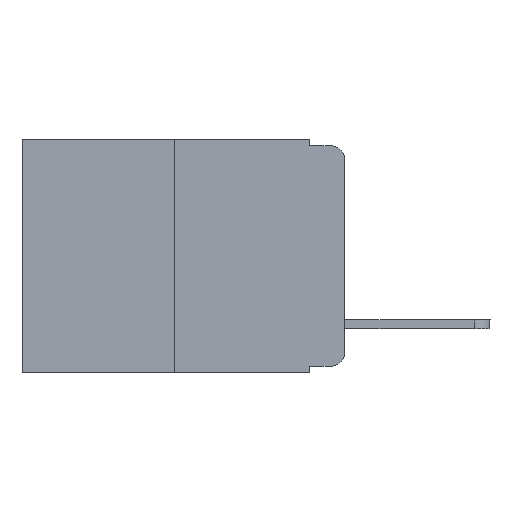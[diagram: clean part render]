
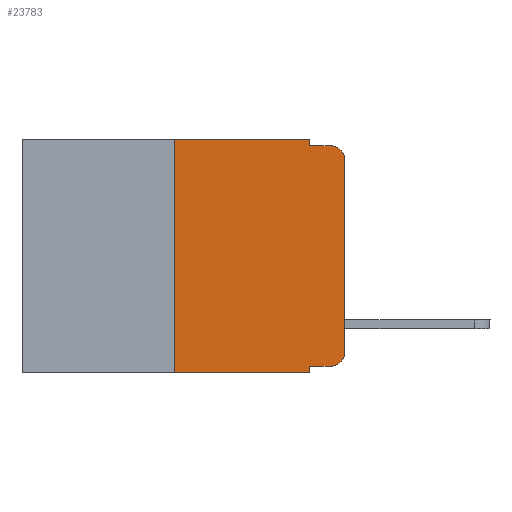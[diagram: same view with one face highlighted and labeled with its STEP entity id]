
A CAD part, left-side view. The second image highlights one B-rep face of the part: STEP entity #23783.
In plain terms, the highlighted planar face has unit normal (-1, 0, 0).
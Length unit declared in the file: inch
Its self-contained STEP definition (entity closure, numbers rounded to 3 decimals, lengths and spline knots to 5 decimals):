
#122 = CARTESIAN_POINT ( 'NONE',  ( 0., 0.25, -0.343 ) ) ;
#177 = ORIENTED_EDGE ( 'NONE', *, *, #20102, .F. ) ;
#269 = AXIS2_PLACEMENT_3D ( 'NONE', #5759, #7558, #11463 ) ;
#439 = DIRECTION ( 'NONE',  ( 0., 0., -1. ) ) ;
#513 = CARTESIAN_POINT ( 'NONE',  ( 0., 0.051, 0. ) ) ;
#537 = DIRECTION ( 'NONE',  ( 0., -1., 0. ) ) ;
#1593 = VECTOR ( 'NONE', #10630, 39.37008 ) ;
#1850 = VERTEX_POINT ( 'NONE', #20672 ) ;
#1998 = DIRECTION ( 'NONE',  ( 0., 0., -1. ) ) ;
#2379 = VERTEX_POINT ( 'NONE', #18623 ) ;
#2406 = ORIENTED_EDGE ( 'NONE', *, *, #16903, .T. ) ;
#3853 = VERTEX_POINT ( 'NONE', #6978 ) ;
#4086 = LINE ( 'NONE', #17225, #21577 ) ;
#4166 = ORIENTED_EDGE ( 'NONE', *, *, #22114, .F. ) ;
#4589 = LINE ( 'NONE', #5526, #17070 ) ;
#4627 = DIRECTION ( 'NONE',  ( 0., -1., 0. ) ) ;
#4696 = EDGE_LOOP ( 'NONE', ( #5741, #11026, #177, #17013, #11236, #5435, #10007, #4166, #2406, #10488 ) ) ;
#5435 = ORIENTED_EDGE ( 'NONE', *, *, #19730, .F. ) ;
#5526 = CARTESIAN_POINT ( 'NONE',  ( 0., 0., 0. ) ) ;
#5741 = ORIENTED_EDGE ( 'NONE', *, *, #14274, .T. ) ;
#5759 = CARTESIAN_POINT ( 'NONE',  ( 0., 0.473, 0. ) ) ;
#5960 = DIRECTION ( 'NONE',  ( 0., 0., -1. ) ) ;
#6978 = CARTESIAN_POINT ( 'NONE',  ( 0., 0.051, -0.343 ) ) ;
#7090 = VERTEX_POINT ( 'NONE', #17525 ) ;
#7213 = VERTEX_POINT ( 'NONE', #21332 ) ;
#7558 = DIRECTION ( 'NONE',  ( 1., 0., 0. ) ) ;
#7773 = LINE ( 'NONE', #12404, #1593 ) ;
#7803 = PLANE ( 'NONE',  #269 ) ;
#8147 = CARTESIAN_POINT ( 'NONE',  ( 0., 0.473, 0. ) ) ;
#8758 = LINE ( 'NONE', #8147, #18013 ) ;
#8973 = DIRECTION ( 'NONE',  ( -1., 0., 0. ) ) ;
#9135 = LINE ( 'NONE', #17227, #18108 ) ;
#9773 = CIRCLE ( 'NONE', #20121, 0.02 ) ;
#10007 = ORIENTED_EDGE ( 'NONE', *, *, #23182, .T. ) ;
#10488 = ORIENTED_EDGE ( 'NONE', *, *, #12250, .T. ) ;
#10630 = DIRECTION ( 'NONE',  ( 0., 0., 1. ) ) ;
#11026 = ORIENTED_EDGE ( 'NONE', *, *, #17869, .T. ) ;
#11236 = ORIENTED_EDGE ( 'NONE', *, *, #18863, .F. ) ;
#11435 = DIRECTION ( 'NONE',  ( -1., 0., 0. ) ) ;
#11463 = DIRECTION ( 'NONE',  ( 0., 0., -1. ) ) ;
#11502 = CARTESIAN_POINT ( 'NONE',  ( 0., 0.051, 0. ) ) ;
#11730 = DIRECTION ( 'NONE',  ( 0., -1., 0. ) ) ;
#12250 = EDGE_CURVE ( 'NONE', #2379, #14583, #9773, .T. ) ;
#12393 = CARTESIAN_POINT ( 'NONE',  ( 0., 0.051, -0.333 ) ) ;
#12404 = CARTESIAN_POINT ( 'NONE',  ( 0., 0.25, 0. ) ) ;
#13252 = VERTEX_POINT ( 'NONE', #513 ) ;
#13514 = CARTESIAN_POINT ( 'NONE',  ( 0., 0.02, -0.01 ) ) ;
#14272 = CARTESIAN_POINT ( 'NONE',  ( 0., 0.02, -0.03 ) ) ;
#14274 = EDGE_CURVE ( 'NONE', #14583, #7213, #4589, .T. ) ;
#14583 = VERTEX_POINT ( 'NONE', #19643 ) ;
#14585 = CIRCLE ( 'NONE', #17061, 0.02 ) ;
#14718 = DIRECTION ( 'NONE',  ( 0., 0., 1. ) ) ;
#14923 = VECTOR ( 'NONE', #537, 39.37008 ) ;
#15267 = LINE ( 'NONE', #11502, #21446 ) ;
#15287 = VECTOR ( 'NONE', #4627, 39.37008 ) ;
#15658 = DIRECTION ( 'NONE',  ( 0., -1., 0. ) ) ;
#16164 = LINE ( 'NONE', #20034, #15287 ) ;
#16903 = EDGE_CURVE ( 'NONE', #18139, #2379, #17539, .T. ) ;
#17013 = ORIENTED_EDGE ( 'NONE', *, *, #20464, .F. ) ;
#17061 = AXIS2_PLACEMENT_3D ( 'NONE', #14272, #8973, #23546 ) ;
#17070 = VECTOR ( 'NONE', #14718, 39.37008 ) ;
#17225 = CARTESIAN_POINT ( 'NONE',  ( 0., 0.473, -0.343 ) ) ;
#17227 = CARTESIAN_POINT ( 'NONE',  ( 0., 0.051, 0. ) ) ;
#17525 = CARTESIAN_POINT ( 'NONE',  ( 0., 0.051, -0.01 ) ) ;
#17539 = LINE ( 'NONE', #22920, #14923 ) ;
#17869 = EDGE_CURVE ( 'NONE', #7213, #22347, #14585, .T. ) ;
#18013 = VECTOR ( 'NONE', #15658, 39.37008 ) ;
#18108 = VECTOR ( 'NONE', #439, 39.37008 ) ;
#18139 = VERTEX_POINT ( 'NONE', #12393 ) ;
#18623 = CARTESIAN_POINT ( 'NONE',  ( 0., 0.02, -0.333 ) ) ;
#18863 = EDGE_CURVE ( 'NONE', #1850, #13252, #8758, .T. ) ;
#19643 = CARTESIAN_POINT ( 'NONE',  ( 0., 0., -0.313 ) ) ;
#19730 = EDGE_CURVE ( 'NONE', #23116, #1850, #7773, .T. ) ;
#20034 = CARTESIAN_POINT ( 'NONE',  ( 0., 0.051, -0.01 ) ) ;
#20102 = EDGE_CURVE ( 'NONE', #7090, #22347, #16164, .T. ) ;
#20121 = AXIS2_PLACEMENT_3D ( 'NONE', #22589, #11435, #5960 ) ;
#20464 = EDGE_CURVE ( 'NONE', #13252, #7090, #15267, .T. ) ;
#20672 = CARTESIAN_POINT ( 'NONE',  ( 0., 0.25, 0. ) ) ;
#21332 = CARTESIAN_POINT ( 'NONE',  ( 0., 0., -0.03 ) ) ;
#21446 = VECTOR ( 'NONE', #1998, 39.37008 ) ;
#21577 = VECTOR ( 'NONE', #11730, 39.37008 ) ;
#22114 = EDGE_CURVE ( 'NONE', #18139, #3853, #9135, .T. ) ;
#22347 = VERTEX_POINT ( 'NONE', #13514 ) ;
#22589 = CARTESIAN_POINT ( 'NONE',  ( 0., 0.02, -0.313 ) ) ;
#22920 = CARTESIAN_POINT ( 'NONE',  ( 0., 0.051, -0.333 ) ) ;
#23026 = FACE_OUTER_BOUND ( 'NONE', #4696, .T. ) ;
#23116 = VERTEX_POINT ( 'NONE', #122 ) ;
#23182 = EDGE_CURVE ( 'NONE', #23116, #3853, #4086, .T. ) ;
#23546 = DIRECTION ( 'NONE',  ( 0., 0., -1. ) ) ;
#23783 = ADVANCED_FACE ( 'NONE', ( #23026 ), #7803, .F. ) ;
